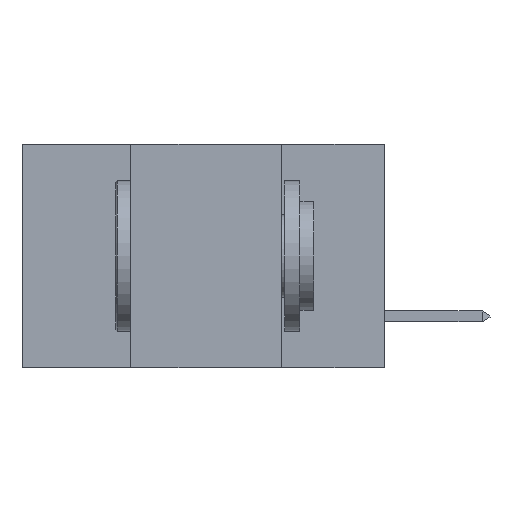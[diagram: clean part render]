
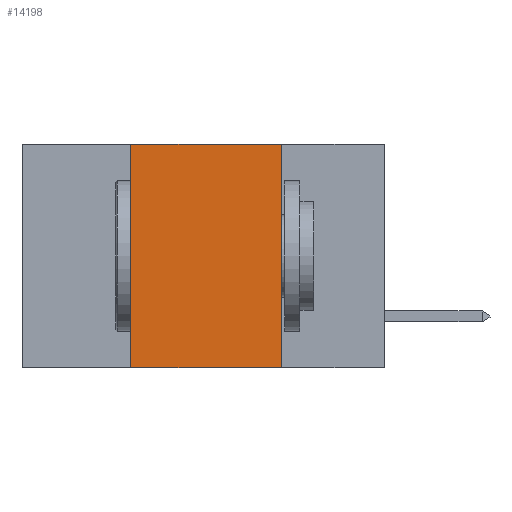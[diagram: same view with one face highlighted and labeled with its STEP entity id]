
A CAD part, left-side view. The second image highlights one B-rep face of the part: STEP entity #14198.
In plain terms, the highlighted planar face has unit normal (-1, 0, 0).
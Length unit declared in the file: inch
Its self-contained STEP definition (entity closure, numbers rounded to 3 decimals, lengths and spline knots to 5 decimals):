
#432 = DIRECTION ( 'NONE',  ( 0., 0., -1. ) ) ;
#829 = VERTEX_POINT ( 'NONE', #21744 ) ;
#1699 = EDGE_LOOP ( 'NONE', ( #11749, #16216, #3692, #17259 ) ) ;
#1969 = VECTOR ( 'NONE', #432, 39.37008 ) ;
#2102 = DIRECTION ( 'NONE',  ( 0., -1., 0. ) ) ;
#2252 = CARTESIAN_POINT ( 'NONE',  ( 0., 0.6, 0. ) ) ;
#2898 = AXIS2_PLACEMENT_3D ( 'NONE', #2252, #20853, #10902 ) ;
#3692 = ORIENTED_EDGE ( 'NONE', *, *, #11892, .F. ) ;
#3985 = LINE ( 'NONE', #4540, #12609 ) ;
#4540 = CARTESIAN_POINT ( 'NONE',  ( 0., 0.6, -0.37 ) ) ;
#5096 = VERTEX_POINT ( 'NONE', #15847 ) ;
#5288 = VECTOR ( 'NONE', #16951, 39.37008 ) ;
#6023 = FACE_OUTER_BOUND ( 'NONE', #1699, .T. ) ;
#6725 = LINE ( 'NONE', #20649, #10774 ) ;
#7076 = LINE ( 'NONE', #20781, #1969 ) ;
#7980 = DIRECTION ( 'NONE',  ( 0., -1., 0. ) ) ;
#10652 = CARTESIAN_POINT ( 'NONE',  ( 0., 0.42, 0. ) ) ;
#10774 = VECTOR ( 'NONE', #2102, 39.37008 ) ;
#10902 = DIRECTION ( 'NONE',  ( 0., 0., -1. ) ) ;
#11749 = ORIENTED_EDGE ( 'NONE', *, *, #14178, .F. ) ;
#11892 = EDGE_CURVE ( 'NONE', #21247, #14800, #18264, .T. ) ;
#12609 = VECTOR ( 'NONE', #7980, 39.37008 ) ;
#14178 = EDGE_CURVE ( 'NONE', #5096, #829, #7076, .T. ) ;
#14198 = ADVANCED_FACE ( 'NONE', ( #6023 ), #19198, .F. ) ;
#14800 = VERTEX_POINT ( 'NONE', #10652 ) ;
#15847 = CARTESIAN_POINT ( 'NONE',  ( 0., 0.17, 0. ) ) ;
#15903 = EDGE_CURVE ( 'NONE', #14800, #5096, #6725, .T. ) ;
#16216 = ORIENTED_EDGE ( 'NONE', *, *, #15903, .F. ) ;
#16951 = DIRECTION ( 'NONE',  ( 0., 0., 1. ) ) ;
#17259 = ORIENTED_EDGE ( 'NONE', *, *, #17492, .T. ) ;
#17492 = EDGE_CURVE ( 'NONE', #21247, #829, #3985, .T. ) ;
#18264 = LINE ( 'NONE', #20174, #5288 ) ;
#19198 = PLANE ( 'NONE',  #2898 ) ;
#20174 = CARTESIAN_POINT ( 'NONE',  ( 0., 0.42, 0. ) ) ;
#20649 = CARTESIAN_POINT ( 'NONE',  ( 0., 0.6, 0. ) ) ;
#20781 = CARTESIAN_POINT ( 'NONE',  ( 0., 0.17, 0. ) ) ;
#20853 = DIRECTION ( 'NONE',  ( 1., 0., 0. ) ) ;
#21060 = CARTESIAN_POINT ( 'NONE',  ( 0., 0.42, -0.37 ) ) ;
#21247 = VERTEX_POINT ( 'NONE', #21060 ) ;
#21744 = CARTESIAN_POINT ( 'NONE',  ( 0., 0.17, -0.37 ) ) ;
